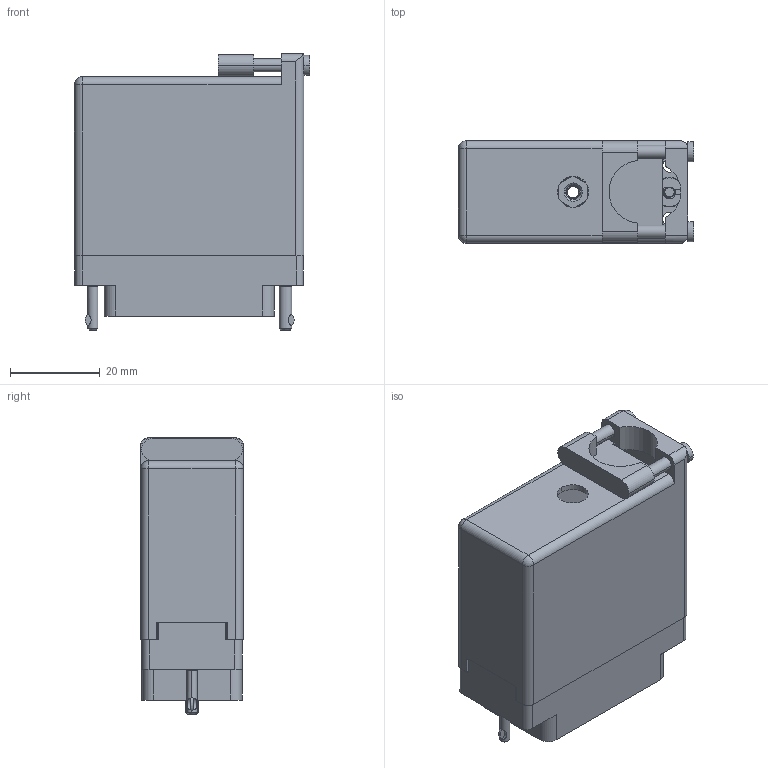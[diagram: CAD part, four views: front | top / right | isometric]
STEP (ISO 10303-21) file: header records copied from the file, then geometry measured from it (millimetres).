
FILE_DESCRIPTION (( 'STEP AP203' ), '1' );
FILE_NAME ('519-036-000-362.STEP', '2020-03-11T16:06:17', ( '' ), ( '' ), 'SwSTEP 2.0', 'SolidWorks 2016', '' );
FILE_SCHEMA (( 'CONFIG_CONTROL_DESIGN' ));
Length unit declared in the file: inch
Products named in the file (7): 516-230-001_Metal - 038 Top Entry; 516-252-035-100_516-252-035-100; 516-252-021-102_038; 516-222-038-102_039; 519 Plug Insulator_036; 519-036-000-362; 516-222-038-102_038
Assembly tree (7 placements, depth 2):
  519-036-000-362
    519 Plug Insulator_036
    516-252-035-100_516-252-035-100
    516-252-021-102_038  x2
    516-222-038-102_038
    516-222-038-102_039
    516-230-001_Metal - 038 Top Entry
Bounding box: 52.27 x 22.83 x 61.42 mm (x, y, z)
Volume: 18569.4 mm3; surface area: 26626.9 mm2
Topology: 7 solids, 7 shells, 1155 faces, 3287 edges, 2166 vertices
Faces by surface type: plane 703, cylinder 358, cone 46, bspline 42, torus 4, sphere 2
Entity records: 44057 total; most frequent: CARTESIAN_POINT 13724, ORIENTED_EDGE 6390, DIRECTION 5989, EDGE_CURVE 3195, VECTOR 2141, LINE 2141, VERTEX_POINT 2106, AXIS2_PLACEMENT_3D 1924
